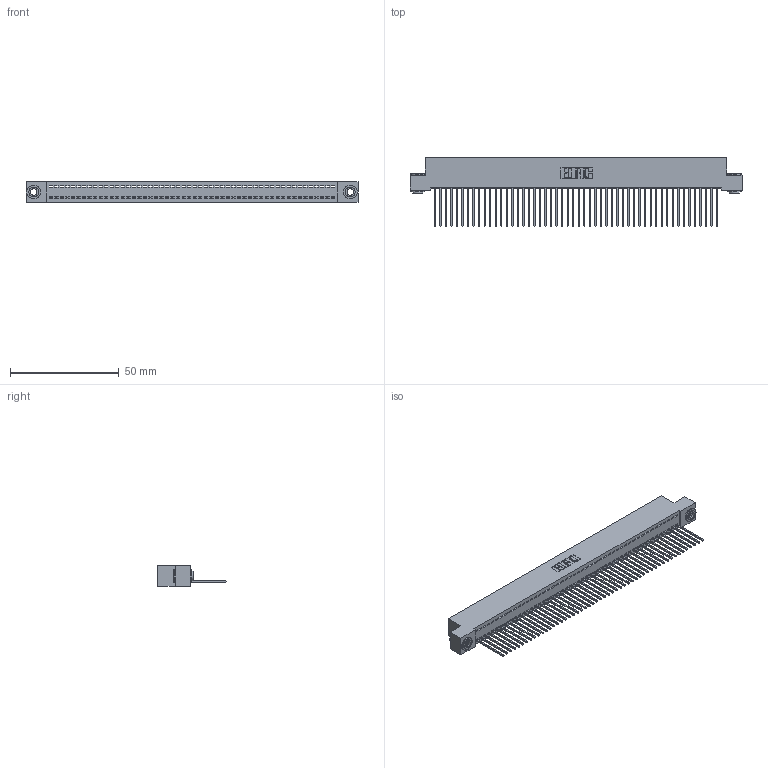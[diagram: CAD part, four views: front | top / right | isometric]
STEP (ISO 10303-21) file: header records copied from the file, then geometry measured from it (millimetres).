
FILE_DESCRIPTION (( 'STEP AP203' ), '1' );
FILE_NAME ('342-052-542-103.STEP', '2018-08-12T22:08:13', ( '' ), ( '' ), 'SwSTEP 2.0', 'SolidWorks 2016', '' );
FILE_SCHEMA (( 'CONFIG_CONTROL_DESIGN' ));
Length unit declared in the file: inch
Products named in the file (4): 342 Part_.156 TH; 345-292-001_345-293-142; 342-250-002_345-250-002-102; 342-052-542-103
Assembly tree (55 placements, depth 2):
  342-052-542-103
    342 Part_.156 TH
    345-292-001_345-293-142  x52
    342-250-002_345-250-002-102  x2
Bounding box: 152.4 x 31.63 x 9.4 mm (x, y, z)
Volume: 13537.8 mm3; surface area: 20998.1 mm2
Topology: 55 solids, 55 shells, 3164 faces, 9527 edges, 6278 vertices
Faces by surface type: plane 2260, cylinder 896, cone 8
Entity records: 31032 total; most frequent: CARTESIAN_POINT 5329, ORIENTED_EDGE 5310, DIRECTION 4509, EDGE_CURVE 2655, LINE 2503, VECTOR 2503, VERTEX_POINT 1766, AXIS2_PLACEMENT_3D 1003
